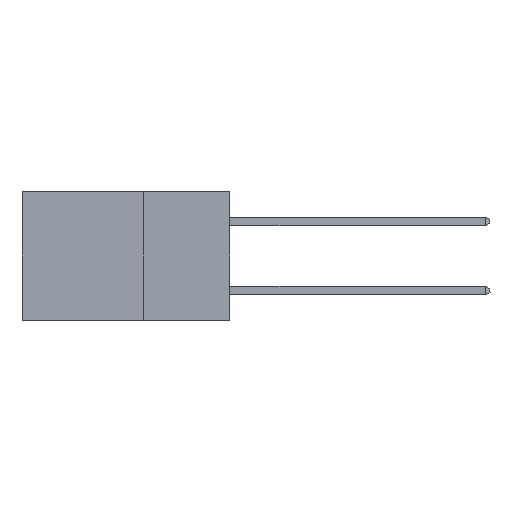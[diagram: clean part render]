
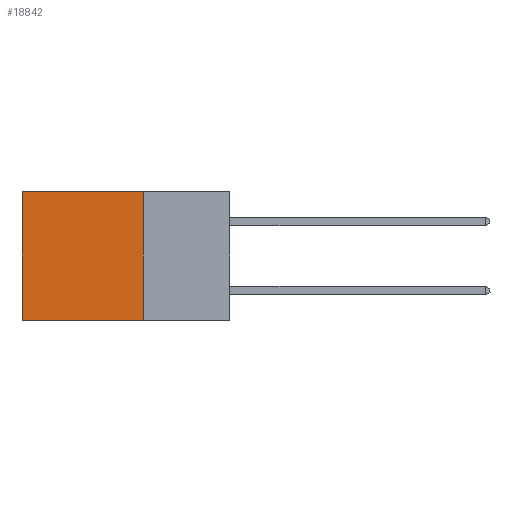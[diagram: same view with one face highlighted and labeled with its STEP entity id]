
A CAD part, left-side view. The second image highlights one B-rep face of the part: STEP entity #18842.
In plain terms, the highlighted planar face has unit normal (-1, 0, 0).
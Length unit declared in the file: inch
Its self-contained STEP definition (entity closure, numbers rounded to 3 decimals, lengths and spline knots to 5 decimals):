
#426 = CARTESIAN_POINT ( 'NONE',  ( 0.298, 0.25, -0.37 ) ) ;
#802 = DIRECTION ( 'NONE',  ( 0., 0., -1. ) ) ;
#847 = CARTESIAN_POINT ( 'NONE',  ( 0.298, 0.25, 0. ) ) ;
#1641 = EDGE_CURVE ( 'NONE', #14028, #13065, #2341, .T. ) ;
#2142 = DIRECTION ( 'NONE',  ( 0., 1., 0. ) ) ;
#2341 = LINE ( 'NONE', #11543, #21553 ) ;
#2416 = ORIENTED_EDGE ( 'NONE', *, *, #1641, .F. ) ;
#2943 = FACE_OUTER_BOUND ( 'NONE', #14299, .T. ) ;
#2967 = EDGE_CURVE ( 'NONE', #14028, #21641, #7115, .T. ) ;
#3222 = LINE ( 'NONE', #3994, #20855 ) ;
#3994 = CARTESIAN_POINT ( 'NONE',  ( 0.298, 0.6, 0. ) ) ;
#4156 = VERTEX_POINT ( 'NONE', #19467 ) ;
#5577 = PLANE ( 'NONE',  #14079 ) ;
#6252 = ORIENTED_EDGE ( 'NONE', *, *, #2967, .T. ) ;
#6384 = EDGE_CURVE ( 'NONE', #21641, #4156, #3222, .T. ) ;
#7115 = LINE ( 'NONE', #847, #20748 ) ;
#9179 = LINE ( 'NONE', #426, #12147 ) ;
#10753 = DIRECTION ( 'NONE',  ( 0., 0., -1. ) ) ;
#10798 = ORIENTED_EDGE ( 'NONE', *, *, #10948, .F. ) ;
#10948 = EDGE_CURVE ( 'NONE', #13065, #4156, #9179, .T. ) ;
#11543 = CARTESIAN_POINT ( 'NONE',  ( 0.298, 0.25, 0. ) ) ;
#12147 = VECTOR ( 'NONE', #2142, 39.37008 ) ;
#13065 = VERTEX_POINT ( 'NONE', #13227 ) ;
#13227 = CARTESIAN_POINT ( 'NONE',  ( 0.298, 0.25, -0.37 ) ) ;
#14028 = VERTEX_POINT ( 'NONE', #21766 ) ;
#14079 = AXIS2_PLACEMENT_3D ( 'NONE', #17535, #20930, #10753 ) ;
#14299 = EDGE_LOOP ( 'NONE', ( #15765, #10798, #2416, #6252 ) ) ;
#14748 = DIRECTION ( 'NONE',  ( 0., 0., -1. ) ) ;
#15765 = ORIENTED_EDGE ( 'NONE', *, *, #6384, .T. ) ;
#17535 = CARTESIAN_POINT ( 'NONE',  ( 0.298, 0.25, 0. ) ) ;
#18842 = ADVANCED_FACE ( 'NONE', ( #2943 ), #5577, .F. ) ;
#19032 = CARTESIAN_POINT ( 'NONE',  ( 0.298, 0.6, 0. ) ) ;
#19467 = CARTESIAN_POINT ( 'NONE',  ( 0.298, 0.6, -0.37 ) ) ;
#20748 = VECTOR ( 'NONE', #21422, 39.37008 ) ;
#20855 = VECTOR ( 'NONE', #802, 39.37008 ) ;
#20930 = DIRECTION ( 'NONE',  ( 1., 0., 0. ) ) ;
#21422 = DIRECTION ( 'NONE',  ( 0., 1., 0. ) ) ;
#21553 = VECTOR ( 'NONE', #14748, 39.37008 ) ;
#21641 = VERTEX_POINT ( 'NONE', #19032 ) ;
#21766 = CARTESIAN_POINT ( 'NONE',  ( 0.298, 0.25, 0. ) ) ;
